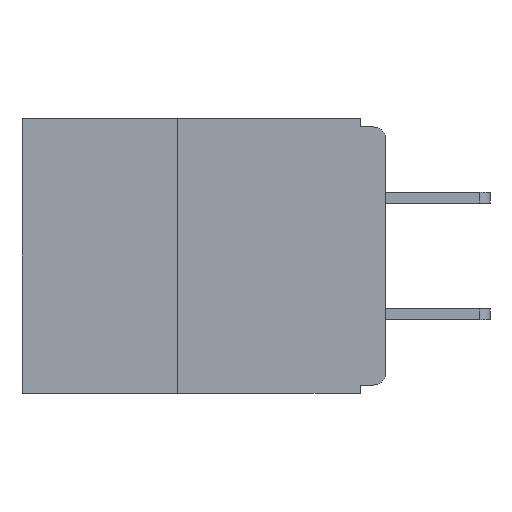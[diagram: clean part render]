
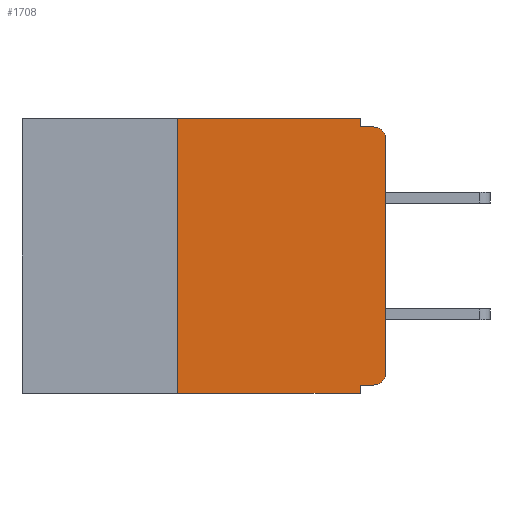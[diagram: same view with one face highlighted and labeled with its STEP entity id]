
A CAD part, left-side view. The second image highlights one B-rep face of the part: STEP entity #1708.
In plain terms, the highlighted planar face has unit normal (-1, 0, 0).
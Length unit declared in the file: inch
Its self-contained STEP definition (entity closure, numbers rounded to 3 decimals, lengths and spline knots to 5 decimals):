
#157 = ORIENTED_EDGE ( 'NONE', *, *, #6928, .F. ) ;
#290 = DIRECTION ( 'NONE',  ( 0., 0., -1. ) ) ;
#366 = EDGE_LOOP ( 'NONE', ( #8956, #1600, #1551, #2571, #759, #1399, #5153, #1924, #157, #1921 ) ) ;
#759 = ORIENTED_EDGE ( 'NONE', *, *, #7570, .F. ) ;
#860 = CARTESIAN_POINT ( 'NONE',  ( 0., 0., 0. ) ) ;
#898 = DIRECTION ( 'NONE',  ( 0., 0., -1. ) ) ;
#1000 = VERTEX_POINT ( 'NONE', #7609 ) ;
#1135 = CARTESIAN_POINT ( 'NONE',  ( 0., 0.031, 0. ) ) ;
#1300 = LINE ( 'NONE', #13488, #6503 ) ;
#1399 = ORIENTED_EDGE ( 'NONE', *, *, #5542, .F. ) ;
#1551 = ORIENTED_EDGE ( 'NONE', *, *, #9458, .F. ) ;
#1600 = ORIENTED_EDGE ( 'NONE', *, *, #11251, .T. ) ;
#1628 = LINE ( 'NONE', #860, #6817 ) ;
#1708 = ADVANCED_FACE ( 'NONE', ( #1779 ), #12362, .F. ) ;
#1779 = FACE_OUTER_BOUND ( 'NONE', #366, .T. ) ;
#1921 = ORIENTED_EDGE ( 'NONE', *, *, #9796, .T. ) ;
#1924 = ORIENTED_EDGE ( 'NONE', *, *, #9075, .F. ) ;
#2067 = VERTEX_POINT ( 'NONE', #10578 ) ;
#2274 = VERTEX_POINT ( 'NONE', #6310 ) ;
#2290 = DIRECTION ( 'NONE',  ( 0., -1., 0. ) ) ;
#2319 = VECTOR ( 'NONE', #13309, 39.37008 ) ;
#2571 = ORIENTED_EDGE ( 'NONE', *, *, #11709, .F. ) ;
#3484 = VECTOR ( 'NONE', #6378, 39.37008 ) ;
#3494 = LINE ( 'NONE', #10615, #11594 ) ;
#3584 = VERTEX_POINT ( 'NONE', #1135 ) ;
#3591 = VECTOR ( 'NONE', #2290, 39.37008 ) ;
#3701 = CARTESIAN_POINT ( 'NONE',  ( 0., 0.437, 0. ) ) ;
#3704 = DIRECTION ( 'NONE',  ( 0., -1., 0. ) ) ;
#3883 = CARTESIAN_POINT ( 'NONE',  ( 0., 0.031, -0.01 ) ) ;
#4081 = VERTEX_POINT ( 'NONE', #11279 ) ;
#4215 = CARTESIAN_POINT ( 'NONE',  ( 0., 0., -0.025 ) ) ;
#4523 = AXIS2_PLACEMENT_3D ( 'NONE', #6971, #10283, #4910 ) ;
#4821 = LINE ( 'NONE', #11271, #12929 ) ;
#4910 = DIRECTION ( 'NONE',  ( 0., 0., -1. ) ) ;
#4977 = DIRECTION ( 'NONE',  ( -1., 0., 0. ) ) ;
#5153 = ORIENTED_EDGE ( 'NONE', *, *, #7373, .T. ) ;
#5542 = EDGE_CURVE ( 'NONE', #4081, #1000, #4821, .T. ) ;
#5884 = CARTESIAN_POINT ( 'NONE',  ( 0., 0.031, -0.33 ) ) ;
#6131 = CARTESIAN_POINT ( 'NONE',  ( 0., 0.437, -0.33 ) ) ;
#6310 = CARTESIAN_POINT ( 'NONE',  ( 0., 0.015, -0.32 ) ) ;
#6378 = DIRECTION ( 'NONE',  ( 0., -1., 0. ) ) ;
#6493 = DIRECTION ( 'NONE',  ( -1., 0., 0. ) ) ;
#6503 = VECTOR ( 'NONE', #898, 39.37008 ) ;
#6672 = VERTEX_POINT ( 'NONE', #13560 ) ;
#6817 = VECTOR ( 'NONE', #13396, 39.37008 ) ;
#6928 = EDGE_CURVE ( 'NONE', #2274, #12196, #3494, .T. ) ;
#6971 = CARTESIAN_POINT ( 'NONE',  ( 0., 0.437, 0. ) ) ;
#7028 = VECTOR ( 'NONE', #3704, 39.37008 ) ;
#7373 = EDGE_CURVE ( 'NONE', #4081, #9183, #11897, .T. ) ;
#7570 = EDGE_CURVE ( 'NONE', #1000, #3584, #12049, .T. ) ;
#7609 = CARTESIAN_POINT ( 'NONE',  ( 0., 0.25, 0. ) ) ;
#8956 = ORIENTED_EDGE ( 'NONE', *, *, #11694, .T. ) ;
#9075 = EDGE_CURVE ( 'NONE', #12196, #9183, #10374, .T. ) ;
#9183 = VERTEX_POINT ( 'NONE', #13447 ) ;
#9303 = CIRCLE ( 'NONE', #13318, 0.015 ) ;
#9458 = EDGE_CURVE ( 'NONE', #13405, #2067, #12980, .T. ) ;
#9796 = EDGE_CURVE ( 'NONE', #2274, #6672, #10170, .T. ) ;
#10170 = CIRCLE ( 'NONE', #10410, 0.015 ) ;
#10283 = DIRECTION ( 'NONE',  ( 1., 0., 0. ) ) ;
#10374 = LINE ( 'NONE', #5884, #2319 ) ;
#10410 = AXIS2_PLACEMENT_3D ( 'NONE', #11336, #4977, #12391 ) ;
#10415 = DIRECTION ( 'NONE',  ( 0., 1., 0. ) ) ;
#10578 = CARTESIAN_POINT ( 'NONE',  ( 0., 0.015, -0.01 ) ) ;
#10615 = CARTESIAN_POINT ( 'NONE',  ( 0., 0., -0.32 ) ) ;
#11212 = DIRECTION ( 'NONE',  ( 0., 0., 1. ) ) ;
#11251 = EDGE_CURVE ( 'NONE', #12963, #2067, #9303, .T. ) ;
#11271 = CARTESIAN_POINT ( 'NONE',  ( 0., 0.25, -0.33 ) ) ;
#11279 = CARTESIAN_POINT ( 'NONE',  ( 0., 0.25, -0.33 ) ) ;
#11336 = CARTESIAN_POINT ( 'NONE',  ( 0., 0.015, -0.305 ) ) ;
#11594 = VECTOR ( 'NONE', #10415, 39.37008 ) ;
#11694 = EDGE_CURVE ( 'NONE', #6672, #12963, #1628, .T. ) ;
#11709 = EDGE_CURVE ( 'NONE', #3584, #13405, #1300, .T. ) ;
#11897 = LINE ( 'NONE', #6131, #3484 ) ;
#12049 = LINE ( 'NONE', #3701, #7028 ) ;
#12196 = VERTEX_POINT ( 'NONE', #13480 ) ;
#12362 = PLANE ( 'NONE',  #4523 ) ;
#12391 = DIRECTION ( 'NONE',  ( 0., 0., -1. ) ) ;
#12726 = CARTESIAN_POINT ( 'NONE',  ( 0., 0., -0.01 ) ) ;
#12863 = CARTESIAN_POINT ( 'NONE',  ( 0., 0.015, -0.025 ) ) ;
#12929 = VECTOR ( 'NONE', #11212, 39.37008 ) ;
#12963 = VERTEX_POINT ( 'NONE', #4215 ) ;
#12980 = LINE ( 'NONE', #12726, #3591 ) ;
#13309 = DIRECTION ( 'NONE',  ( 0., 0., -1. ) ) ;
#13318 = AXIS2_PLACEMENT_3D ( 'NONE', #12863, #6493, #290 ) ;
#13396 = DIRECTION ( 'NONE',  ( 0., 0., 1. ) ) ;
#13405 = VERTEX_POINT ( 'NONE', #3883 ) ;
#13447 = CARTESIAN_POINT ( 'NONE',  ( 0., 0.031, -0.33 ) ) ;
#13480 = CARTESIAN_POINT ( 'NONE',  ( 0., 0.031, -0.32 ) ) ;
#13488 = CARTESIAN_POINT ( 'NONE',  ( 0., 0.031, 0. ) ) ;
#13560 = CARTESIAN_POINT ( 'NONE',  ( 0., 0., -0.305 ) ) ;
